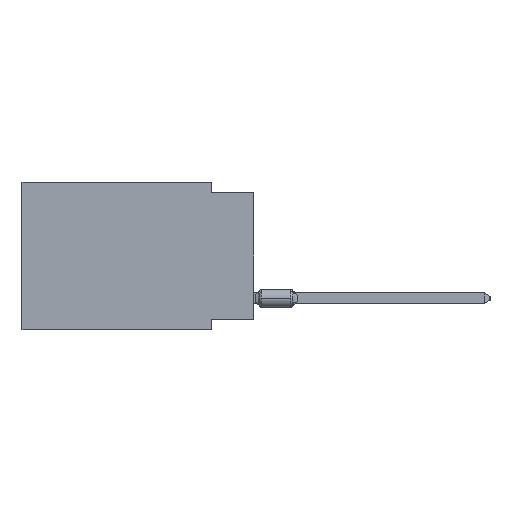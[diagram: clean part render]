
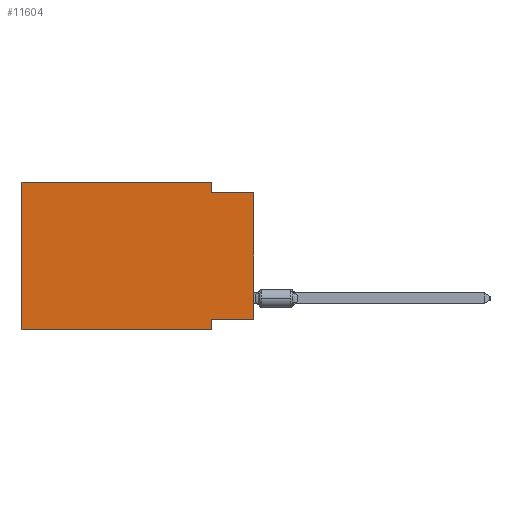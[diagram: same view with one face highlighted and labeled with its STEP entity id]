
A CAD part, left-side view. The second image highlights one B-rep face of the part: STEP entity #11604.
In plain terms, the highlighted planar face has unit normal (-1, 0, 0).
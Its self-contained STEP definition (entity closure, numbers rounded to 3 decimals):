
#824 = ORIENTED_EDGE ( 'NONE', *, *, #32846, .F. ) ;
#1415 = CARTESIAN_POINT ( 'NONE',  ( 0., 0., -8.255 ) ) ;
#1646 = DIRECTION ( 'NONE',  ( 1., 0., 0. ) ) ;
#3679 = LINE ( 'NONE', #28087, #80353 ) ;
#6991 = VERTEX_POINT ( 'NONE', #38449 ) ;
#9074 = LINE ( 'NONE', #113525, #68470 ) ;
#9306 = CARTESIAN_POINT ( 'NONE',  ( 0., 13.97, 0. ) ) ;
#9469 = ORIENTED_EDGE ( 'NONE', *, *, #84495, .F. ) ;
#10444 = ORIENTED_EDGE ( 'NONE', *, *, #42448, .F. ) ;
#11604 = ADVANCED_FACE ( 'NONE', ( #53342 ), #26635, .F. ) ;
#16076 = ORIENTED_EDGE ( 'NONE', *, *, #62092, .F. ) ;
#19075 = CARTESIAN_POINT ( 'NONE',  ( 0., 13.97, 0. ) ) ;
#19583 = VERTEX_POINT ( 'NONE', #35291 ) ;
#22267 = EDGE_CURVE ( 'NONE', #86679, #6991, #9074, .T. ) ;
#22846 = CARTESIAN_POINT ( 'NONE',  ( 0., 0., -0.635 ) ) ;
#24378 = LINE ( 'NONE', #24943, #53634 ) ;
#24943 = CARTESIAN_POINT ( 'NONE',  ( 0., 2.54, 0. ) ) ;
#26635 = PLANE ( 'NONE',  #33602 ) ;
#26667 = CARTESIAN_POINT ( 'NONE',  ( 0., 2.54, -8.255 ) ) ;
#27122 = DIRECTION ( 'NONE',  ( 0., 1., 0. ) ) ;
#28087 = CARTESIAN_POINT ( 'NONE',  ( 0., 2.54, -8.89 ) ) ;
#29403 = CARTESIAN_POINT ( 'NONE',  ( 0., 2.54, -8.89 ) ) ;
#32630 = EDGE_CURVE ( 'NONE', #19583, #55790, #53415, .T. ) ;
#32846 = EDGE_CURVE ( 'NONE', #86679, #114125, #38665, .T. ) ;
#33602 = AXIS2_PLACEMENT_3D ( 'NONE', #19075, #1646, #80030 ) ;
#35291 = CARTESIAN_POINT ( 'NONE',  ( 0., 13.97, -8.89 ) ) ;
#35356 = DIRECTION ( 'NONE',  ( 0., 0., -1. ) ) ;
#38449 = CARTESIAN_POINT ( 'NONE',  ( 0., 0., -0.635 ) ) ;
#38640 = VECTOR ( 'NONE', #99626, 1000. ) ;
#38649 = DIRECTION ( 'NONE',  ( 0., -1., 0. ) ) ;
#38665 = LINE ( 'NONE', #82788, #40740 ) ;
#40273 = VERTEX_POINT ( 'NONE', #29403 ) ;
#40740 = VECTOR ( 'NONE', #27122, 1000. ) ;
#41801 = EDGE_CURVE ( 'NONE', #19583, #40273, #63092, .T. ) ;
#42448 = EDGE_CURVE ( 'NONE', #55790, #84517, #95354, .T. ) ;
#42548 = LINE ( 'NONE', #22846, #103225 ) ;
#50393 = EDGE_LOOP ( 'NONE', ( #73914, #16076, #9469, #10444, #75958, #63082, #63908, #824 ) ) ;
#51464 = DIRECTION ( 'NONE',  ( 0., 0., 1. ) ) ;
#51836 = VECTOR ( 'NONE', #38649, 1000. ) ;
#53342 = FACE_OUTER_BOUND ( 'NONE', #50393, .T. ) ;
#53415 = LINE ( 'NONE', #9306, #75890 ) ;
#53634 = VECTOR ( 'NONE', #35356, 1000. ) ;
#55790 = VERTEX_POINT ( 'NONE', #89340 ) ;
#62092 = EDGE_CURVE ( 'NONE', #78707, #6991, #42548, .T. ) ;
#63082 = ORIENTED_EDGE ( 'NONE', *, *, #41801, .T. ) ;
#63092 = LINE ( 'NONE', #71803, #38640 ) ;
#63908 = ORIENTED_EDGE ( 'NONE', *, *, #93032, .F. ) ;
#68470 = VECTOR ( 'NONE', #51464, 1000. ) ;
#69668 = DIRECTION ( 'NONE',  ( 0., 0., 1. ) ) ;
#71803 = CARTESIAN_POINT ( 'NONE',  ( 0., 13.97, -8.89 ) ) ;
#73914 = ORIENTED_EDGE ( 'NONE', *, *, #22267, .T. ) ;
#75890 = VECTOR ( 'NONE', #69668, 1000. ) ;
#75958 = ORIENTED_EDGE ( 'NONE', *, *, #32630, .F. ) ;
#78707 = VERTEX_POINT ( 'NONE', #110725 ) ;
#80030 = DIRECTION ( 'NONE',  ( 0., 0., -1. ) ) ;
#80353 = VECTOR ( 'NONE', #82607, 1000. ) ;
#82607 = DIRECTION ( 'NONE',  ( 0., 0., -1. ) ) ;
#82788 = CARTESIAN_POINT ( 'NONE',  ( 0., 0., -8.255 ) ) ;
#84495 = EDGE_CURVE ( 'NONE', #84517, #78707, #24378, .T. ) ;
#84517 = VERTEX_POINT ( 'NONE', #95164 ) ;
#86679 = VERTEX_POINT ( 'NONE', #1415 ) ;
#89340 = CARTESIAN_POINT ( 'NONE',  ( 0., 13.97, 0. ) ) ;
#89760 = CARTESIAN_POINT ( 'NONE',  ( 0., 13.97, 0. ) ) ;
#93032 = EDGE_CURVE ( 'NONE', #114125, #40273, #3679, .T. ) ;
#95164 = CARTESIAN_POINT ( 'NONE',  ( 0., 2.54, 0. ) ) ;
#95354 = LINE ( 'NONE', #89760, #51836 ) ;
#99626 = DIRECTION ( 'NONE',  ( 0., -1., 0. ) ) ;
#103225 = VECTOR ( 'NONE', #111031, 1000. ) ;
#110725 = CARTESIAN_POINT ( 'NONE',  ( 0., 2.54, -0.635 ) ) ;
#111031 = DIRECTION ( 'NONE',  ( 0., -1., 0. ) ) ;
#113525 = CARTESIAN_POINT ( 'NONE',  ( 0., 0., 0. ) ) ;
#114125 = VERTEX_POINT ( 'NONE', #26667 ) ;
